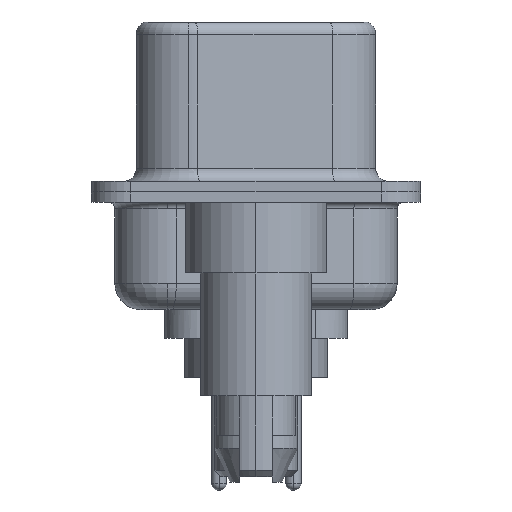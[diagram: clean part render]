
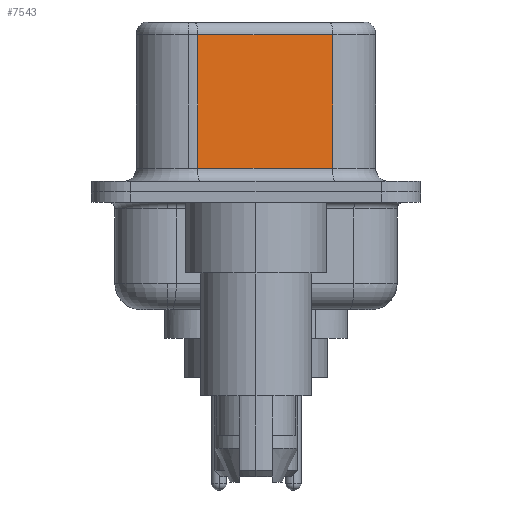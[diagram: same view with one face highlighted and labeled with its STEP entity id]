
A CAD part, left-side view. The second image highlights one B-rep face of the part: STEP entity #7543.
In plain terms, the highlighted planar face has unit normal (-0.985, -0.174, 0).
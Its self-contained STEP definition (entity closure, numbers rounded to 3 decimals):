
#155 = VERTEX_POINT ( 'NONE', #893 ) ;
#179 = ORIENTED_EDGE ( 'NONE', *, *, #16809, .F. ) ;
#203 = CARTESIAN_POINT ( 'NONE',  ( 4.585, -2.927, 0.9 ) ) ;
#345 = EDGE_CURVE ( 'NONE', #4215, #155, #16256, .T. ) ;
#522 = ORIENTED_EDGE ( 'NONE', *, *, #16808, .T. ) ;
#893 = CARTESIAN_POINT ( 'NONE',  ( 3.675, 2.233, 0.9 ) ) ;
#1029 = VECTOR ( 'NONE', #12550, 1000. ) ;
#1934 = ORIENTED_EDGE ( 'NONE', *, *, #345, .T. ) ;
#1964 = DIRECTION ( 'NONE',  ( 0.174, -0.985, 0. ) ) ;
#3955 = VECTOR ( 'NONE', #15740, 1000. ) ;
#4215 = VERTEX_POINT ( 'NONE', #9427 ) ;
#4292 = CARTESIAN_POINT ( 'NONE',  ( 4.585, -2.927, 0.9 ) ) ;
#4660 = CARTESIAN_POINT ( 'NONE',  ( 4.585, -2.927, 6.52 ) ) ;
#5051 = VERTEX_POINT ( 'NONE', #4292 ) ;
#6548 = EDGE_LOOP ( 'NONE', ( #179, #13217, #1934, #522 ) ) ;
#7349 = FACE_OUTER_BOUND ( 'NONE', #6548, .T. ) ;
#7543 = ADVANCED_FACE ( 'NONE', ( #7349 ), #20834, .F. ) ;
#7656 = AXIS2_PLACEMENT_3D ( 'NONE', #4660, #18272, #8310 ) ;
#8310 = DIRECTION ( 'NONE',  ( -0.174, 0.985, 0. ) ) ;
#9427 = CARTESIAN_POINT ( 'NONE',  ( 3.675, 2.233, 6.02 ) ) ;
#10844 = CARTESIAN_POINT ( 'NONE',  ( 4.585, -2.927, 6.02 ) ) ;
#11897 = DIRECTION ( 'NONE',  ( 0., 0., -1. ) ) ;
#12011 = CARTESIAN_POINT ( 'NONE',  ( 4.585, -2.927, 6.02 ) ) ;
#12550 = DIRECTION ( 'NONE',  ( -0.174, 0.985, 0. ) ) ;
#13137 = VECTOR ( 'NONE', #1964, 1000. ) ;
#13192 = VERTEX_POINT ( 'NONE', #12011 ) ;
#13217 = ORIENTED_EDGE ( 'NONE', *, *, #16366, .T. ) ;
#14004 = CARTESIAN_POINT ( 'NONE',  ( 4.585, -2.927, 6.52 ) ) ;
#14194 = LINE ( 'NONE', #203, #13137 ) ;
#14746 = LINE ( 'NONE', #10844, #1029 ) ;
#15687 = VECTOR ( 'NONE', #11897, 1000. ) ;
#15740 = DIRECTION ( 'NONE',  ( 0., 0., -1. ) ) ;
#16256 = LINE ( 'NONE', #20015, #15687 ) ;
#16366 = EDGE_CURVE ( 'NONE', #13192, #4215, #14746, .T. ) ;
#16808 = EDGE_CURVE ( 'NONE', #155, #5051, #14194, .T. ) ;
#16809 = EDGE_CURVE ( 'NONE', #13192, #5051, #17739, .T. ) ;
#17739 = LINE ( 'NONE', #14004, #3955 ) ;
#18272 = DIRECTION ( 'NONE',  ( 0.985, 0.174, 0. ) ) ;
#20015 = CARTESIAN_POINT ( 'NONE',  ( 3.675, 2.233, 6.52 ) ) ;
#20834 = PLANE ( 'NONE',  #7656 ) ;
